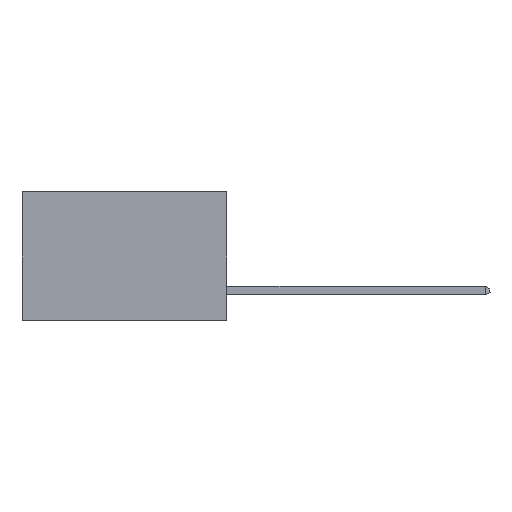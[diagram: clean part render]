
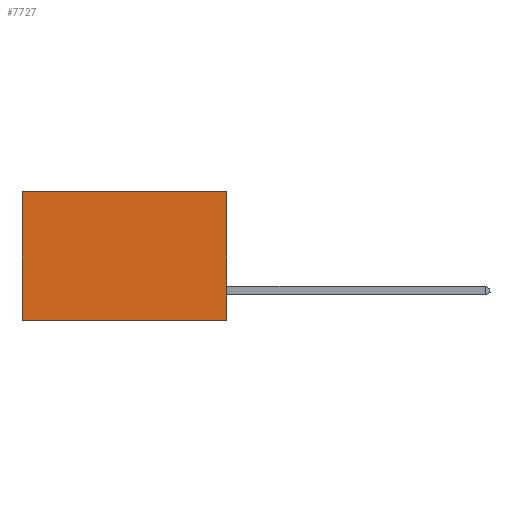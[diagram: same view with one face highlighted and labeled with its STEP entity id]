
A CAD part, left-side view. The second image highlights one B-rep face of the part: STEP entity #7727.
In plain terms, the highlighted planar face has unit normal (-1, 0, 0).
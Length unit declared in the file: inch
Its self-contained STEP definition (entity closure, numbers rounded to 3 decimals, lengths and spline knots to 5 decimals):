
#453 = DIRECTION ( 'NONE',  ( 0., 0., -1. ) ) ;
#550 = VERTEX_POINT ( 'NONE', #14694 ) ;
#564 = DIRECTION ( 'NONE',  ( 0., 1., 0. ) ) ;
#665 = CARTESIAN_POINT ( 'NONE',  ( 0.277, 0., 0. ) ) ;
#1727 = LINE ( 'NONE', #665, #3215 ) ;
#1892 = VERTEX_POINT ( 'NONE', #25176 ) ;
#2411 = VECTOR ( 'NONE', #453, 39.37008 ) ;
#2491 = EDGE_CURVE ( 'NONE', #11166, #18887, #3150, .T. ) ;
#2857 = ORIENTED_EDGE ( 'NONE', *, *, #2491, .T. ) ;
#3150 = LINE ( 'NONE', #6828, #2411 ) ;
#3215 = VECTOR ( 'NONE', #564, 39.37008 ) ;
#3757 = ORIENTED_EDGE ( 'NONE', *, *, #28617, .F. ) ;
#6828 = CARTESIAN_POINT ( 'NONE',  ( 0.277, 0.59, -0.37 ) ) ;
#7727 = ADVANCED_FACE ( 'NONE', ( #9693 ), #18886, .F. ) ;
#8018 = EDGE_CURVE ( 'NONE', #550, #11166, #1727, .T. ) ;
#8248 = LINE ( 'NONE', #13372, #24149 ) ;
#9693 = FACE_OUTER_BOUND ( 'NONE', #11192, .T. ) ;
#10551 = CARTESIAN_POINT ( 'NONE',  ( 0.277, 0., -0.37 ) ) ;
#11166 = VERTEX_POINT ( 'NONE', #16131 ) ;
#11192 = EDGE_LOOP ( 'NONE', ( #2857, #3757, #17705, #13198 ) ) ;
#12578 = VECTOR ( 'NONE', #21895, 39.37008 ) ;
#13198 = ORIENTED_EDGE ( 'NONE', *, *, #8018, .T. ) ;
#13372 = CARTESIAN_POINT ( 'NONE',  ( 0.277, 0., -0.37 ) ) ;
#14694 = CARTESIAN_POINT ( 'NONE',  ( 0.277, 0., 0. ) ) ;
#15118 = EDGE_CURVE ( 'NONE', #550, #1892, #24490, .T. ) ;
#16131 = CARTESIAN_POINT ( 'NONE',  ( 0.277, 0.59, 0. ) ) ;
#16410 = AXIS2_PLACEMENT_3D ( 'NONE', #18854, #18585, #18428 ) ;
#17705 = ORIENTED_EDGE ( 'NONE', *, *, #15118, .F. ) ;
#18428 = DIRECTION ( 'NONE',  ( 0., 0., -1. ) ) ;
#18585 = DIRECTION ( 'NONE',  ( 1., 0., 0. ) ) ;
#18854 = CARTESIAN_POINT ( 'NONE',  ( 0.277, 0., -0.37 ) ) ;
#18886 = PLANE ( 'NONE',  #16410 ) ;
#18887 = VERTEX_POINT ( 'NONE', #24618 ) ;
#20124 = DIRECTION ( 'NONE',  ( 0., 1., 0. ) ) ;
#21895 = DIRECTION ( 'NONE',  ( 0., 0., -1. ) ) ;
#24149 = VECTOR ( 'NONE', #20124, 39.37008 ) ;
#24490 = LINE ( 'NONE', #10551, #12578 ) ;
#24618 = CARTESIAN_POINT ( 'NONE',  ( 0.277, 0.59, -0.37 ) ) ;
#25176 = CARTESIAN_POINT ( 'NONE',  ( 0.277, 0., -0.37 ) ) ;
#28617 = EDGE_CURVE ( 'NONE', #1892, #18887, #8248, .T. ) ;
